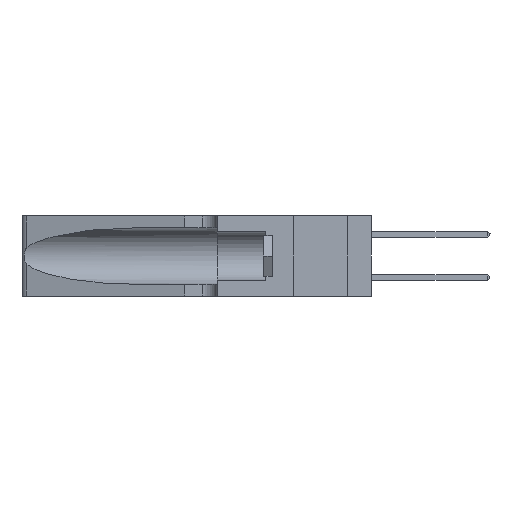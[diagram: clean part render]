
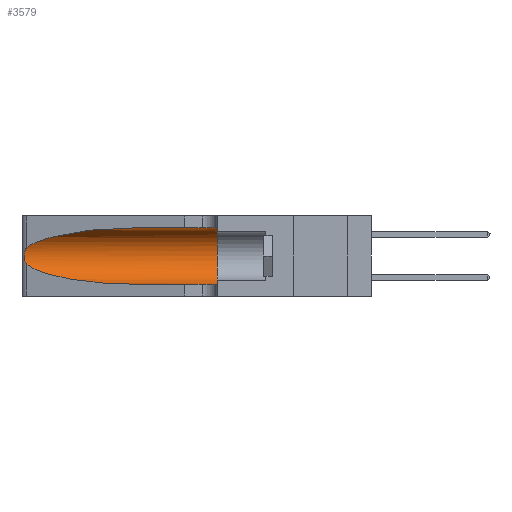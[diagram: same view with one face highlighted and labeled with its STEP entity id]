
A CAD part, left-side view. The second image highlights one B-rep face of the part: STEP entity #3579.
In plain terms, the highlighted cylindrical face has radius 3.308 mm (diameter 6.617 mm), a partial arc.
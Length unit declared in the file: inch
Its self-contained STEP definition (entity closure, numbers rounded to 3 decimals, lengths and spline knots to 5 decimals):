
#224 = CARTESIAN_POINT ( 'NONE',  ( 0.25555, 1.22993, 0.14849 ) ) ;
#534 = VERTEX_POINT ( 'NONE', #18817 ) ;
#2100 = CARTESIAN_POINT ( 'NONE',  ( 0.2373, 1.15595, 0.08982 ) ) ;
#2295 = CARTESIAN_POINT ( 'NONE',  ( 0.25639, 1.23186, 0.15144 ) ) ;
#2381 = VERTEX_POINT ( 'NONE', #5382 ) ;
#2497 = CARTESIAN_POINT ( 'NONE',  ( 0.25555, 1.22994, 0.2215 ) ) ;
#2572 = CARTESIAN_POINT ( 'NONE',  ( 0.1305, 1.61858, 0.185 ) ) ;
#2885 = EDGE_LOOP ( 'NONE', ( #25927, #8011, #3827, #25114, #7367, #24320 ) ) ;
#2972 = VERTEX_POINT ( 'NONE', #18304 ) ;
#3579 = ADVANCED_FACE ( 'NONE', ( #24162 ), #10002, .F. ) ;
#3827 = ORIENTED_EDGE ( 'NONE', *, *, #15681, .T. ) ;
#4872 = CARTESIAN_POINT ( 'NONE',  ( 0.25787, 1.23484, 0.2124 ) ) ;
#5382 = CARTESIAN_POINT ( 'NONE',  ( 0.25487, 1.22718, 0.22369 ) ) ;
#5551 = CARTESIAN_POINT ( 'NONE',  ( 0.1305, 1.61858, 0.05475 ) ) ;
#5760 = DIRECTION ( 'NONE',  ( 0., -1., 0. ) ) ;
#5941 = AXIS2_PLACEMENT_3D ( 'NONE', #2572, #12427, #12216 ) ;
#6262 = VERTEX_POINT ( 'NONE', #15559 ) ;
#6735 = CARTESIAN_POINT ( 'NONE',  ( 0.18966, 0.96281, 0.31525 ) ) ;
#7113 =( BOUNDED_CURVE ( )  B_SPLINE_CURVE ( 3, ( #18542, #6735, #23338, #13488 ),
 .UNSPECIFIED., .F., .F. ) 
 B_SPLINE_CURVE_WITH_KNOTS ( ( 4, 4 ),
 ( 1.5708, 2.84003 ),
 .UNSPECIFIED. ) 
 CURVE ( )  GEOMETRIC_REPRESENTATION_ITEM ( )  RATIONAL_B_SPLINE_CURVE ( ( 1., 0.87, 0.87, 1. ) ) 
 REPRESENTATION_ITEM ( '' )  );
#7367 = ORIENTED_EDGE ( 'NONE', *, *, #8940, .F. ) ;
#7391 = CARTESIAN_POINT ( 'NONE',  ( 0.25856, 1.23593, 0.16098 ) ) ;
#8011 = ORIENTED_EDGE ( 'NONE', *, *, #25900, .T. ) ;
#8448 = DIRECTION ( 'NONE',  ( 0., 1., 0. ) ) ;
#8940 = EDGE_CURVE ( 'NONE', #15283, #534, #12545, .T. ) ;
#9661 = CARTESIAN_POINT ( 'NONE',  ( 0.25487, 1.22718, 0.22369 ) ) ;
#9762 = CARTESIAN_POINT ( 'NONE',  ( 0.26075, 1.23896, 0.178 ) ) ;
#9987 = CARTESIAN_POINT ( 'NONE',  ( 0.1305, 0.35, 0.31525 ) ) ;
#10002 = CYLINDRICAL_SURFACE ( 'NONE', #5941, 0.13025 ) ;
#11591 = AXIS2_PLACEMENT_3D ( 'NONE', #29843, #8448, #24963 ) ;
#11643 = CARTESIAN_POINT ( 'NONE',  ( 0.1305, 0.72297, 0.05475 ) ) ;
#11833 = CARTESIAN_POINT ( 'NONE',  ( 0.26075, 1.23896, 0.19203 ) ) ;
#12139 = CARTESIAN_POINT ( 'NONE',  ( 0.26017, 1.23833, 0.17102 ) ) ;
#12216 = DIRECTION ( 'NONE',  ( 0., 0., -1. ) ) ;
#12427 = DIRECTION ( 'NONE',  ( 0., -1., 0. ) ) ;
#12545 = CIRCLE ( 'NONE', #11591, 0.13025 ) ;
#13488 = CARTESIAN_POINT ( 'NONE',  ( 0.25487, 1.22718, 0.22369 ) ) ;
#14734 = VECTOR ( 'NONE', #21371, 39.37008 ) ;
#15283 = VERTEX_POINT ( 'NONE', #9987 ) ;
#15559 = CARTESIAN_POINT ( 'NONE',  ( 0.1305, 0.72297, 0.05475 ) ) ;
#15637 = EDGE_CURVE ( 'NONE', #2972, #15283, #19210, .T. ) ;
#15681 = EDGE_CURVE ( 'NONE', #22401, #6262, #16215, .T. ) ;
#16215 =( BOUNDED_CURVE ( )  B_SPLINE_CURVE ( 3, ( #28172, #2100, #21070, #11643 ),
 .UNSPECIFIED., .F., .F. ) 
 B_SPLINE_CURVE_WITH_KNOTS ( ( 4, 4 ),
 ( 3.44316, 4.71239 ),
 .UNSPECIFIED. ) 
 CURVE ( )  GEOMETRIC_REPRESENTATION_ITEM ( )  RATIONAL_B_SPLINE_CURVE ( ( 1., 0.87, 0.87, 1. ) ) 
 REPRESENTATION_ITEM ( '' )  );
#16584 = CARTESIAN_POINT ( 'NONE',  ( 0.25639, 1.23184, 0.21858 ) ) ;
#16594 = B_SPLINE_CURVE_WITH_KNOTS ( 'NONE', 3,
 ( #9661, #2497, #16584, #4872, #21472, #21574, #11833, #9762, #12139, #7391, #26388, #2295, #224, #16793 ),
 .UNSPECIFIED., .F., .F.,
 ( 4, 2, 2, 2, 2, 2, 4 ),
 ( 0., 0.00027, 0.00053, 0.00107, 0.0016, 0.00187, 0.00214 ),
 .UNSPECIFIED. ) ;
#16793 = CARTESIAN_POINT ( 'NONE',  ( 0.25487, 1.22718, 0.14631 ) ) ;
#17265 = EDGE_CURVE ( 'NONE', #6262, #534, #19461, .T. ) ;
#17593 = VECTOR ( 'NONE', #5760, 39.37008 ) ;
#18304 = CARTESIAN_POINT ( 'NONE',  ( 0.1305, 0.72297, 0.31525 ) ) ;
#18542 = CARTESIAN_POINT ( 'NONE',  ( 0.1305, 0.72297, 0.31525 ) ) ;
#18817 = CARTESIAN_POINT ( 'NONE',  ( 0.1305, 0.35, 0.05475 ) ) ;
#19210 = LINE ( 'NONE', #23683, #14734 ) ;
#19461 = LINE ( 'NONE', #5551, #17593 ) ;
#21070 = CARTESIAN_POINT ( 'NONE',  ( 0.18966, 0.96281, 0.05475 ) ) ;
#21371 = DIRECTION ( 'NONE',  ( 0., -1., 0. ) ) ;
#21472 = CARTESIAN_POINT ( 'NONE',  ( 0.25854, 1.2359, 0.20912 ) ) ;
#21574 = CARTESIAN_POINT ( 'NONE',  ( 0.26018, 1.23835, 0.19895 ) ) ;
#21635 = EDGE_CURVE ( 'NONE', #2972, #2381, #7113, .T. ) ;
#22401 = VERTEX_POINT ( 'NONE', #23204 ) ;
#23204 = CARTESIAN_POINT ( 'NONE',  ( 0.25487, 1.22718, 0.14631 ) ) ;
#23338 = CARTESIAN_POINT ( 'NONE',  ( 0.2373, 1.15595, 0.28018 ) ) ;
#23683 = CARTESIAN_POINT ( 'NONE',  ( 0.1305, 1.61858, 0.31525 ) ) ;
#24162 = FACE_OUTER_BOUND ( 'NONE', #2885, .T. ) ;
#24320 = ORIENTED_EDGE ( 'NONE', *, *, #15637, .F. ) ;
#24963 = DIRECTION ( 'NONE',  ( 0., 0., 1. ) ) ;
#25114 = ORIENTED_EDGE ( 'NONE', *, *, #17265, .T. ) ;
#25900 = EDGE_CURVE ( 'NONE', #2381, #22401, #16594, .T. ) ;
#25927 = ORIENTED_EDGE ( 'NONE', *, *, #21635, .T. ) ;
#26388 = CARTESIAN_POINT ( 'NONE',  ( 0.25789, 1.23486, 0.15765 ) ) ;
#28172 = CARTESIAN_POINT ( 'NONE',  ( 0.25487, 1.22718, 0.14631 ) ) ;
#29843 = CARTESIAN_POINT ( 'NONE',  ( 0.1305, 0.35, 0.185 ) ) ;
